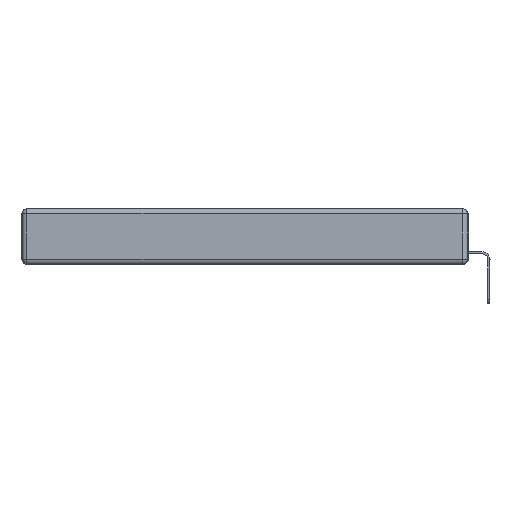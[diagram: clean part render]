
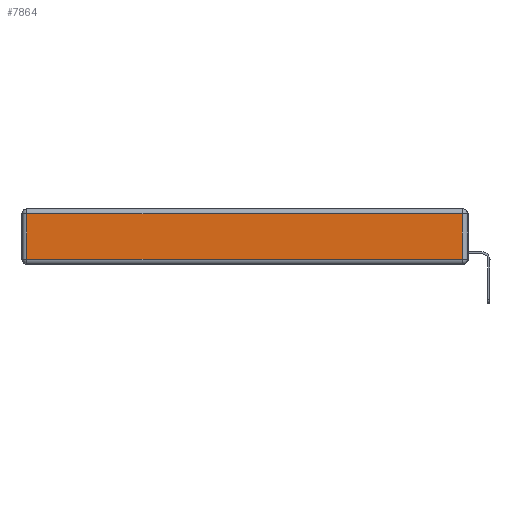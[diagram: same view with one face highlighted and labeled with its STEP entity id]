
A CAD part, left-side view. The second image highlights one B-rep face of the part: STEP entity #7864.
In plain terms, the highlighted planar face has unit normal (-1, 0, 0).
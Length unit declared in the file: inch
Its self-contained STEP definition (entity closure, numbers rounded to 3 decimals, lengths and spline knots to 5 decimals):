
#1773 = VERTEX_POINT ( 'NONE', #21387 ) ;
#5115 = DIRECTION ( 'NONE',  ( 0., 0., -1. ) ) ;
#6892 = ORIENTED_EDGE ( 'NONE', *, *, #15404, .T. ) ;
#7519 = DIRECTION ( 'NONE',  ( 0., 1., 0. ) ) ;
#7864 = ADVANCED_FACE ( 'NONE', ( #24934 ), #15599, .T. ) ;
#7885 = LINE ( 'NONE', #19019, #24110 ) ;
#8229 = DIRECTION ( 'NONE',  ( 0., -1., 0. ) ) ;
#8284 = VECTOR ( 'NONE', #5115, 39.37008 ) ;
#9335 = AXIS2_PLACEMENT_3D ( 'NONE', #21531, #15684, #12032 ) ;
#9982 = VERTEX_POINT ( 'NONE', #13659 ) ;
#10589 = LINE ( 'NONE', #19910, #24454 ) ;
#10648 = VECTOR ( 'NONE', #17579, 39.37008 ) ;
#11847 = ORIENTED_EDGE ( 'NONE', *, *, #23461, .T. ) ;
#12032 = DIRECTION ( 'NONE',  ( 0., 0., 1. ) ) ;
#12119 = ORIENTED_EDGE ( 'NONE', *, *, #20629, .T. ) ;
#12206 = CARTESIAN_POINT ( 'NONE',  ( 0., 0.03, -0.03 ) ) ;
#12598 = CARTESIAN_POINT ( 'NONE',  ( 0., 2.72, -0.313 ) ) ;
#13659 = CARTESIAN_POINT ( 'NONE',  ( 0., 0.03, -0.313 ) ) ;
#14037 = VERTEX_POINT ( 'NONE', #12598 ) ;
#14399 = ORIENTED_EDGE ( 'NONE', *, *, #15048, .T. ) ;
#15048 = EDGE_CURVE ( 'NONE', #14037, #9982, #10589, .T. ) ;
#15404 = EDGE_CURVE ( 'NONE', #15743, #1773, #7885, .T. ) ;
#15599 = PLANE ( 'NONE',  #9335 ) ;
#15684 = DIRECTION ( 'NONE',  ( -1., 0., 0. ) ) ;
#15743 = VERTEX_POINT ( 'NONE', #12206 ) ;
#16363 = LINE ( 'NONE', #23963, #8284 ) ;
#17579 = DIRECTION ( 'NONE',  ( 0., 0., 1. ) ) ;
#19019 = CARTESIAN_POINT ( 'NONE',  ( 0., 2.75, -0.03 ) ) ;
#19910 = CARTESIAN_POINT ( 'NONE',  ( 0., 0., -0.313 ) ) ;
#19986 = LINE ( 'NONE', #24742, #10648 ) ;
#20629 = EDGE_CURVE ( 'NONE', #9982, #15743, #19986, .T. ) ;
#21387 = CARTESIAN_POINT ( 'NONE',  ( 0., 2.72, -0.03 ) ) ;
#21531 = CARTESIAN_POINT ( 'NONE',  ( 0., 0., -0.343 ) ) ;
#23461 = EDGE_CURVE ( 'NONE', #1773, #14037, #16363, .T. ) ;
#23963 = CARTESIAN_POINT ( 'NONE',  ( 0., 2.72, -0.343 ) ) ;
#24110 = VECTOR ( 'NONE', #7519, 39.37008 ) ;
#24454 = VECTOR ( 'NONE', #8229, 39.37008 ) ;
#24620 = EDGE_LOOP ( 'NONE', ( #14399, #12119, #6892, #11847 ) ) ;
#24742 = CARTESIAN_POINT ( 'NONE',  ( 0., 0.03, -0.343 ) ) ;
#24934 = FACE_OUTER_BOUND ( 'NONE', #24620, .T. ) ;
